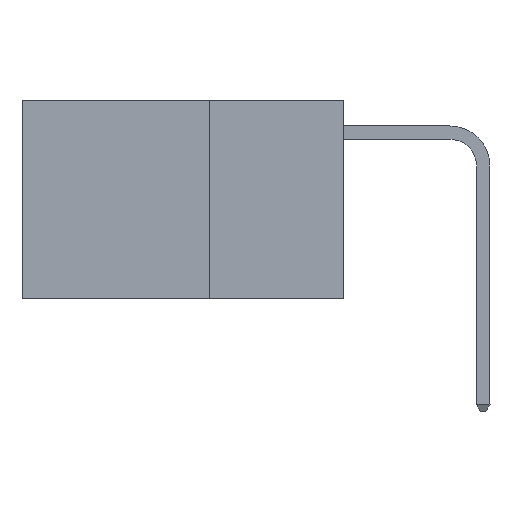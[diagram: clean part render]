
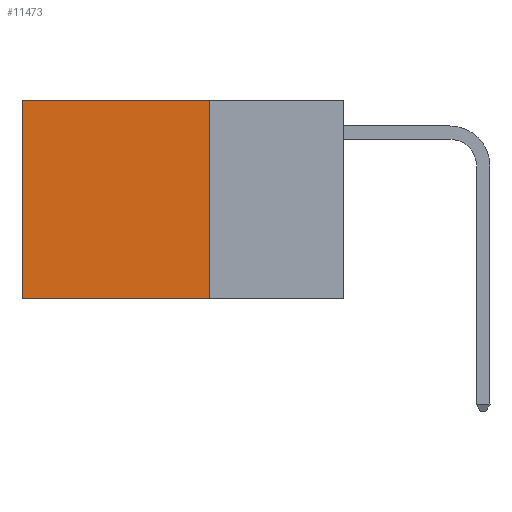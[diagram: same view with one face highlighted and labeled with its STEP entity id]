
A CAD part, left-side view. The second image highlights one B-rep face of the part: STEP entity #11473.
In plain terms, the highlighted planar face has unit normal (-1, 0, 0).
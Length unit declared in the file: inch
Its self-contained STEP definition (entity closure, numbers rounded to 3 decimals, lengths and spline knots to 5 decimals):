
#79 = LINE ( 'NONE', #3331, #14704 ) ;
#2879 = VECTOR ( 'NONE', #8559, 39.37008 ) ;
#3124 = FACE_OUTER_BOUND ( 'NONE', #6127, .T. ) ;
#3168 = VERTEX_POINT ( 'NONE', #17801 ) ;
#3252 = DIRECTION ( 'NONE',  ( 0., 1., 0. ) ) ;
#3331 = CARTESIAN_POINT ( 'NONE',  ( 0.2625, 0.25, 0. ) ) ;
#5629 = EDGE_CURVE ( 'NONE', #3168, #16732, #79, .T. ) ;
#5688 = VECTOR ( 'NONE', #16629, 39.37008 ) ;
#5847 = VERTEX_POINT ( 'NONE', #6448 ) ;
#6127 = EDGE_LOOP ( 'NONE', ( #10138, #20750, #18442, #8674 ) ) ;
#6448 = CARTESIAN_POINT ( 'NONE',  ( 0.2625, 0.6, -0.37 ) ) ;
#7065 = EDGE_CURVE ( 'NONE', #16771, #5847, #23389, .T. ) ;
#7621 = VECTOR ( 'NONE', #11292, 39.37008 ) ;
#8012 = LINE ( 'NONE', #19918, #2879 ) ;
#8559 = DIRECTION ( 'NONE',  ( 0., 0., -1. ) ) ;
#8674 = ORIENTED_EDGE ( 'NONE', *, *, #5629, .T. ) ;
#9871 = CARTESIAN_POINT ( 'NONE',  ( 0.2625, 0.25, 0. ) ) ;
#10138 = ORIENTED_EDGE ( 'NONE', *, *, #15295, .T. ) ;
#11292 = DIRECTION ( 'NONE',  ( 0., 1., 0. ) ) ;
#11342 = CARTESIAN_POINT ( 'NONE',  ( 0.2625, 0.25, -0.37 ) ) ;
#11473 = ADVANCED_FACE ( 'NONE', ( #3124 ), #21285, .F. ) ;
#11727 = DIRECTION ( 'NONE',  ( 0., 0., -1. ) ) ;
#14704 = VECTOR ( 'NONE', #3252, 39.37008 ) ;
#14716 = CARTESIAN_POINT ( 'NONE',  ( 0.2625, 0.6, 0. ) ) ;
#15295 = EDGE_CURVE ( 'NONE', #16732, #5847, #15751, .T. ) ;
#15403 = CARTESIAN_POINT ( 'NONE',  ( 0.2625, 0.6, 0. ) ) ;
#15481 = CARTESIAN_POINT ( 'NONE',  ( 0.2625, 0.25, -0.37 ) ) ;
#15751 = LINE ( 'NONE', #14716, #5688 ) ;
#16629 = DIRECTION ( 'NONE',  ( 0., 0., -1. ) ) ;
#16732 = VERTEX_POINT ( 'NONE', #15403 ) ;
#16771 = VERTEX_POINT ( 'NONE', #15481 ) ;
#16987 = EDGE_CURVE ( 'NONE', #3168, #16771, #8012, .T. ) ;
#17801 = CARTESIAN_POINT ( 'NONE',  ( 0.2625, 0.25, 0. ) ) ;
#18442 = ORIENTED_EDGE ( 'NONE', *, *, #16987, .F. ) ;
#19918 = CARTESIAN_POINT ( 'NONE',  ( 0.2625, 0.25, 0. ) ) ;
#20750 = ORIENTED_EDGE ( 'NONE', *, *, #7065, .F. ) ;
#21285 = PLANE ( 'NONE',  #21397 ) ;
#21397 = AXIS2_PLACEMENT_3D ( 'NONE', #9871, #23218, #11727 ) ;
#23218 = DIRECTION ( 'NONE',  ( 1., 0., 0. ) ) ;
#23389 = LINE ( 'NONE', #11342, #7621 ) ;
